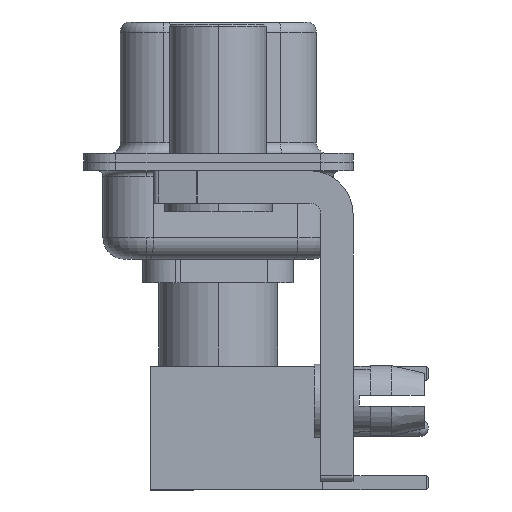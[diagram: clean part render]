
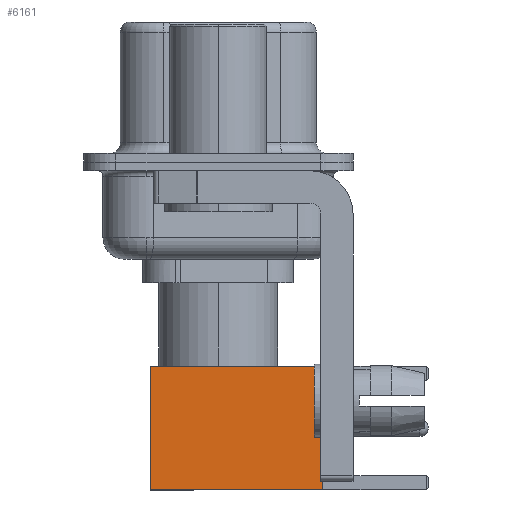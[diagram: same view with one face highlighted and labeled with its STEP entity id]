
A CAD part, left-side view. The second image highlights one B-rep face of the part: STEP entity #6161.
In plain terms, the highlighted face is planar.
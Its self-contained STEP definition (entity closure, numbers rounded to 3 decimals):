
#668 = VERTEX_POINT ( 'NONE', #12838 ) ;
#747 = DIRECTION ( 'NONE',  ( 0., 0., -1. ) ) ;
#952 = EDGE_LOOP ( 'NONE', ( #10381, #1766, #3941, #10557 ) ) ;
#1766 = ORIENTED_EDGE ( 'NONE', *, *, #19966, .T. ) ;
#1845 = CARTESIAN_POINT ( 'NONE',  ( 2.875, 2.875, 0. ) ) ;
#2329 = CARTESIAN_POINT ( 'NONE',  ( 2.875, 2.875, 0. ) ) ;
#2474 = CARTESIAN_POINT ( 'NONE',  ( -2.875, 2.875, 0. ) ) ;
#3755 = FACE_OUTER_BOUND ( 'NONE', #952, .T. ) ;
#3941 = ORIENTED_EDGE ( 'NONE', *, *, #9099, .F. ) ;
#4429 = LINE ( 'NONE', #14396, #18888 ) ;
#6009 = LINE ( 'NONE', #15988, #16030 ) ;
#6161 = ADVANCED_FACE ( 'NONE', ( #3755 ), #17124, .T. ) ;
#6284 = DIRECTION ( 'NONE',  ( -1., 0., 0. ) ) ;
#8220 = AXIS2_PLACEMENT_3D ( 'NONE', #2329, #8914, #20693 ) ;
#8289 = VECTOR ( 'NONE', #10699, 1000. ) ;
#8422 = VERTEX_POINT ( 'NONE', #1845 ) ;
#8580 = EDGE_CURVE ( 'NONE', #9024, #8422, #13681, .T. ) ;
#8914 = DIRECTION ( 'NONE',  ( 0., 1., 0. ) ) ;
#9024 = VERTEX_POINT ( 'NONE', #17190 ) ;
#9099 = EDGE_CURVE ( 'NONE', #668, #15539, #6009, .T. ) ;
#10381 = ORIENTED_EDGE ( 'NONE', *, *, #8580, .T. ) ;
#10557 = ORIENTED_EDGE ( 'NONE', *, *, #16722, .F. ) ;
#10699 = DIRECTION ( 'NONE',  ( 0., 0., -1. ) ) ;
#12639 = DIRECTION ( 'NONE',  ( -1., 0., 0. ) ) ;
#12838 = CARTESIAN_POINT ( 'NONE',  ( -2.875, 2.875, 8. ) ) ;
#13681 = LINE ( 'NONE', #16963, #8289 ) ;
#14396 = CARTESIAN_POINT ( 'NONE',  ( 0., 2.875, 0. ) ) ;
#15539 = VERTEX_POINT ( 'NONE', #2474 ) ;
#15902 = VECTOR ( 'NONE', #12639, 1000. ) ;
#15988 = CARTESIAN_POINT ( 'NONE',  ( -2.875, 2.875, 0. ) ) ;
#16030 = VECTOR ( 'NONE', #747, 1000. ) ;
#16722 = EDGE_CURVE ( 'NONE', #9024, #668, #19599, .T. ) ;
#16963 = CARTESIAN_POINT ( 'NONE',  ( 2.875, 2.875, 0. ) ) ;
#17124 = PLANE ( 'NONE',  #8220 ) ;
#17190 = CARTESIAN_POINT ( 'NONE',  ( 2.875, 2.875, 8. ) ) ;
#18888 = VECTOR ( 'NONE', #6284, 1000. ) ;
#19599 = LINE ( 'NONE', #19701, #15902 ) ;
#19701 = CARTESIAN_POINT ( 'NONE',  ( 0., 2.875, 8. ) ) ;
#19966 = EDGE_CURVE ( 'NONE', #8422, #15539, #4429, .T. ) ;
#20693 = DIRECTION ( 'NONE',  ( 0., 0., 1. ) ) ;
